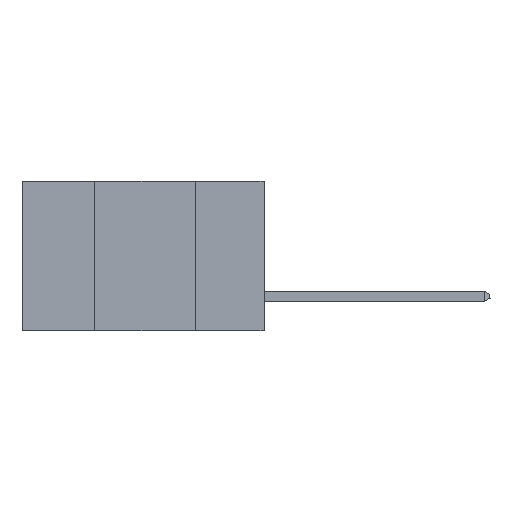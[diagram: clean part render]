
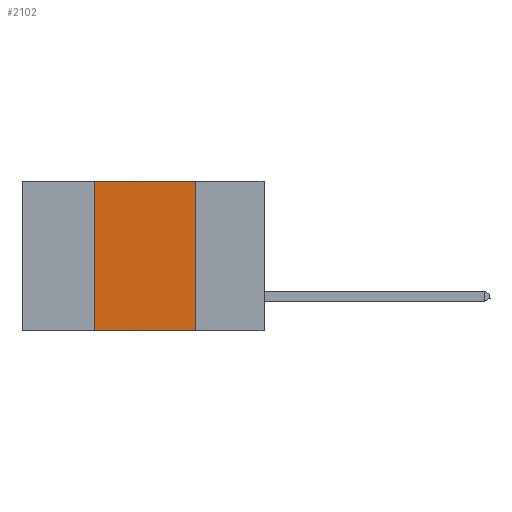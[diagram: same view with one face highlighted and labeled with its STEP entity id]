
A CAD part, left-side view. The second image highlights one B-rep face of the part: STEP entity #2102.
In plain terms, the highlighted planar face has unit normal (-1, 0, 0).
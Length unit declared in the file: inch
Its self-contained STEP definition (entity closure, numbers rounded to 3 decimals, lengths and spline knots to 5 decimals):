
#524 = LINE ( 'NONE', #7889, #7393 ) ;
#891 = CARTESIAN_POINT ( 'NONE',  ( 0., 0.6, 0. ) ) ;
#935 = PLANE ( 'NONE',  #4626 ) ;
#1004 = ORIENTED_EDGE ( 'NONE', *, *, #6503, .F. ) ;
#1293 = ORIENTED_EDGE ( 'NONE', *, *, #14163, .T. ) ;
#1400 = LINE ( 'NONE', #2557, #12758 ) ;
#1970 = DIRECTION ( 'NONE',  ( 1., 0., 0. ) ) ;
#2102 = ADVANCED_FACE ( 'NONE', ( #5113 ), #935, .F. ) ;
#2467 = VECTOR ( 'NONE', #10912, 39.37008 ) ;
#2557 = CARTESIAN_POINT ( 'NONE',  ( 0., 0.42, -0.37 ) ) ;
#3375 = EDGE_LOOP ( 'NONE', ( #13505, #1004, #6440, #1293 ) ) ;
#3587 = VERTEX_POINT ( 'NONE', #6172 ) ;
#4626 = AXIS2_PLACEMENT_3D ( 'NONE', #891, #1970, #13081 ) ;
#4629 = LINE ( 'NONE', #9529, #5287 ) ;
#4977 = CARTESIAN_POINT ( 'NONE',  ( 0., 0.42, 0. ) ) ;
#5113 = FACE_OUTER_BOUND ( 'NONE', #3375, .T. ) ;
#5287 = VECTOR ( 'NONE', #12950, 39.37008 ) ;
#5896 = DIRECTION ( 'NONE',  ( 0., 0., 1. ) ) ;
#6172 = CARTESIAN_POINT ( 'NONE',  ( 0., 0.42, -0.37 ) ) ;
#6440 = ORIENTED_EDGE ( 'NONE', *, *, #6750, .F. ) ;
#6503 = EDGE_CURVE ( 'NONE', #13562, #9321, #524, .T. ) ;
#6750 = EDGE_CURVE ( 'NONE', #3587, #13562, #1400, .T. ) ;
#7393 = VECTOR ( 'NONE', #12321, 39.37008 ) ;
#7552 = CARTESIAN_POINT ( 'NONE',  ( 0., 0.17, -0.37 ) ) ;
#7746 = VERTEX_POINT ( 'NONE', #7552 ) ;
#7889 = CARTESIAN_POINT ( 'NONE',  ( 0., 0.6, 0. ) ) ;
#9321 = VERTEX_POINT ( 'NONE', #12125 ) ;
#9529 = CARTESIAN_POINT ( 'NONE',  ( 0., 0.17, -0.37 ) ) ;
#10128 = EDGE_CURVE ( 'NONE', #9321, #7746, #4629, .T. ) ;
#10912 = DIRECTION ( 'NONE',  ( 0., -1., 0. ) ) ;
#12125 = CARTESIAN_POINT ( 'NONE',  ( 0., 0.17, 0. ) ) ;
#12321 = DIRECTION ( 'NONE',  ( 0., -1., 0. ) ) ;
#12455 = LINE ( 'NONE', #13868, #2467 ) ;
#12758 = VECTOR ( 'NONE', #5896, 39.37008 ) ;
#12950 = DIRECTION ( 'NONE',  ( 0., 0., -1. ) ) ;
#13081 = DIRECTION ( 'NONE',  ( 0., 0., -1. ) ) ;
#13505 = ORIENTED_EDGE ( 'NONE', *, *, #10128, .F. ) ;
#13562 = VERTEX_POINT ( 'NONE', #4977 ) ;
#13868 = CARTESIAN_POINT ( 'NONE',  ( 0., 0.6, -0.37 ) ) ;
#14163 = EDGE_CURVE ( 'NONE', #3587, #7746, #12455, .T. ) ;
